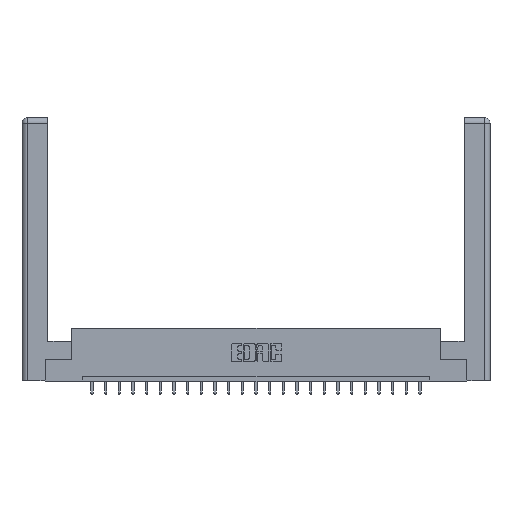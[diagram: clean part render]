
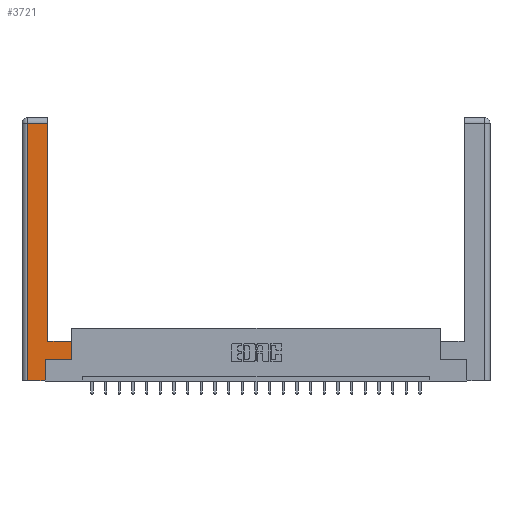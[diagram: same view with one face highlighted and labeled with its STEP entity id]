
A CAD part, top view. The second image highlights one B-rep face of the part: STEP entity #3721.
In plain terms, the highlighted planar face has unit normal (0, 0, 1).
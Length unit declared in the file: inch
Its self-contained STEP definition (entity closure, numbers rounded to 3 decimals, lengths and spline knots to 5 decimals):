
#347 = ORIENTED_EDGE ( 'NONE', *, *, #17100, .T. ) ;
#953 = ORIENTED_EDGE ( 'NONE', *, *, #6323, .T. ) ;
#1275 = CARTESIAN_POINT ( 'NONE',  ( 0.295, 2.94, 0. ) ) ;
#2717 = PLANE ( 'NONE',  #19122 ) ;
#2984 = CARTESIAN_POINT ( 'NONE',  ( 0.0615, 0., 0. ) ) ;
#3234 = VECTOR ( 'NONE', #6112, 39.37008 ) ;
#3308 = CARTESIAN_POINT ( 'NONE',  ( 0.265, 0., 0. ) ) ;
#3412 = VECTOR ( 'NONE', #23217, 39.37008 ) ;
#3590 = DIRECTION ( 'NONE',  ( 0., 1., 0. ) ) ;
#3668 = LINE ( 'NONE', #5457, #16686 ) ;
#3721 = ADVANCED_FACE ( 'NONE', ( #21869 ), #2717, .F. ) ;
#3991 = LINE ( 'NONE', #5131, #3412 ) ;
#4209 = VERTEX_POINT ( 'NONE', #15088 ) ;
#4353 = ORIENTED_EDGE ( 'NONE', *, *, #16276, .T. ) ;
#4610 = DIRECTION ( 'NONE',  ( 0., 1., 0. ) ) ;
#5131 = CARTESIAN_POINT ( 'NONE',  ( 0.0615, 0., 0. ) ) ;
#5457 = CARTESIAN_POINT ( 'NONE',  ( 0.565, 0.245, 0. ) ) ;
#5620 = EDGE_CURVE ( 'NONE', #19696, #11305, #5751, .T. ) ;
#5737 = EDGE_CURVE ( 'NONE', #4209, #23405, #15061, .T. ) ;
#5751 = LINE ( 'NONE', #10356, #7137 ) ;
#6112 = DIRECTION ( 'NONE',  ( 0., 1., 0. ) ) ;
#6323 = EDGE_CURVE ( 'NONE', #19009, #14167, #12466, .T. ) ;
#6422 = LINE ( 'NONE', #19048, #14038 ) ;
#6717 = ORIENTED_EDGE ( 'NONE', *, *, #15259, .T. ) ;
#6740 = VECTOR ( 'NONE', #15933, 39.37008 ) ;
#6862 = DIRECTION ( 'NONE',  ( -1., 0., 0. ) ) ;
#6864 = EDGE_CURVE ( 'NONE', #11305, #14191, #3991, .T. ) ;
#6866 = CARTESIAN_POINT ( 'NONE',  ( 0.0615, 2.94, 0. ) ) ;
#7137 = VECTOR ( 'NONE', #6862, 39.37008 ) ;
#7824 = CARTESIAN_POINT ( 'NONE',  ( 0.295, 3., 0. ) ) ;
#8388 = DIRECTION ( 'NONE',  ( -1., 0., 0. ) ) ;
#9120 = ORIENTED_EDGE ( 'NONE', *, *, #9700, .T. ) ;
#9700 = EDGE_CURVE ( 'NONE', #23405, #19696, #12009, .T. ) ;
#9965 = DIRECTION ( 'NONE',  ( 0., 0., -1. ) ) ;
#10054 = CARTESIAN_POINT ( 'NONE',  ( 0., 0., 0. ) ) ;
#10356 = CARTESIAN_POINT ( 'NONE',  ( 0.0615, 2.94, 0. ) ) ;
#10630 = CARTESIAN_POINT ( 'NONE',  ( 0.295, 0.45, 0. ) ) ;
#10913 = DIRECTION ( 'NONE',  ( 1., 0., 0. ) ) ;
#11305 = VERTEX_POINT ( 'NONE', #6866 ) ;
#11719 = VERTEX_POINT ( 'NONE', #21591 ) ;
#12009 = LINE ( 'NONE', #7824, #3234 ) ;
#12466 = LINE ( 'NONE', #23403, #13611 ) ;
#12628 = ORIENTED_EDGE ( 'NONE', *, *, #5737, .T. ) ;
#13611 = VECTOR ( 'NONE', #3590, 39.37008 ) ;
#13882 = CARTESIAN_POINT ( 'NONE',  ( 0.295, 0.45, 0. ) ) ;
#14038 = VECTOR ( 'NONE', #4610, 39.37008 ) ;
#14131 = CARTESIAN_POINT ( 'NONE',  ( 0.265, 0., 0. ) ) ;
#14167 = VERTEX_POINT ( 'NONE', #15690 ) ;
#14191 = VERTEX_POINT ( 'NONE', #2984 ) ;
#15061 = LINE ( 'NONE', #13882, #19380 ) ;
#15088 = CARTESIAN_POINT ( 'NONE',  ( 0.565, 0.45, 0. ) ) ;
#15259 = EDGE_CURVE ( 'NONE', #14167, #11719, #3668, .T. ) ;
#15323 = DIRECTION ( 'NONE',  ( -1., 0., 0. ) ) ;
#15690 = CARTESIAN_POINT ( 'NONE',  ( 0.265, 0.245, 0. ) ) ;
#15933 = DIRECTION ( 'NONE',  ( 1., 0., 0. ) ) ;
#16276 = EDGE_CURVE ( 'NONE', #14191, #19009, #21224, .T. ) ;
#16686 = VECTOR ( 'NONE', #10913, 39.37008 ) ;
#17100 = EDGE_CURVE ( 'NONE', #11719, #4209, #6422, .T. ) ;
#19009 = VERTEX_POINT ( 'NONE', #14131 ) ;
#19048 = CARTESIAN_POINT ( 'NONE',  ( 0.565, 0.45, 0. ) ) ;
#19122 = AXIS2_PLACEMENT_3D ( 'NONE', #10054, #9965, #15323 ) ;
#19380 = VECTOR ( 'NONE', #8388, 39.37008 ) ;
#19696 = VERTEX_POINT ( 'NONE', #1275 ) ;
#21224 = LINE ( 'NONE', #3308, #6740 ) ;
#21591 = CARTESIAN_POINT ( 'NONE',  ( 0.565, 0.245, 0. ) ) ;
#21702 = EDGE_LOOP ( 'NONE', ( #9120, #22508, #23109, #4353, #953, #6717, #347, #12628 ) ) ;
#21869 = FACE_OUTER_BOUND ( 'NONE', #21702, .T. ) ;
#22508 = ORIENTED_EDGE ( 'NONE', *, *, #5620, .T. ) ;
#23109 = ORIENTED_EDGE ( 'NONE', *, *, #6864, .T. ) ;
#23217 = DIRECTION ( 'NONE',  ( 0., -1., 0. ) ) ;
#23403 = CARTESIAN_POINT ( 'NONE',  ( 0.265, 0.245, 0. ) ) ;
#23405 = VERTEX_POINT ( 'NONE', #10630 ) ;
